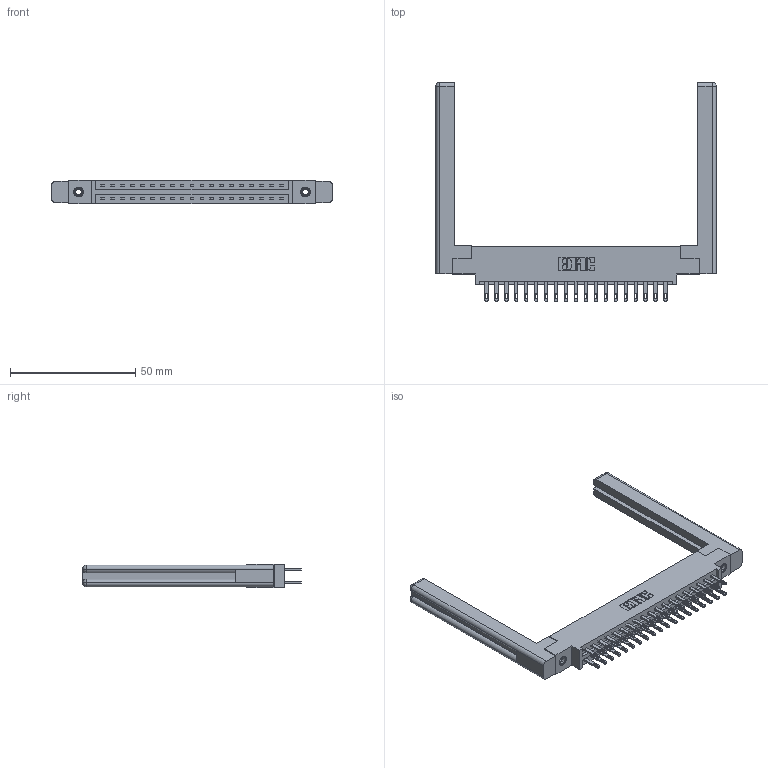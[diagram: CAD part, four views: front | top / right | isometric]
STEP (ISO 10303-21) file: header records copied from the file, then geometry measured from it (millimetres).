
FILE_DESCRIPTION (( 'STEP AP203' ), '1' );
FILE_NAME ('337-038-500-858.STEP', '2019-10-11T11:07:55', ( '' ), ( '' ), 'SwSTEP 2.0', 'SolidWorks 2016', '' );
FILE_SCHEMA (( 'CONFIG_CONTROL_DESIGN' ));
Length unit declared in the file: inch
Products named in the file (5): 337 Part_0.170 Offset - 0.156 Dia-TI; 337-038-500-858; 345-250-001_345-250-001-102; 345-292-001_345-293-100; 307-220-058
Assembly tree (43 placements, depth 2):
  337-038-500-858
    337 Part_0.170 Offset - 0.156 Dia-TI
    345-292-001_345-293-100  x38
    345-250-001_345-250-001-102  x2
    307-220-058  x2
Bounding box: 111.91 x 87.25 x 9.4 mm (x, y, z)
Volume: 18629 mm3; surface area: 18338.5 mm2
Topology: 43 solids, 43 shells, 2160 faces, 6491 edges, 4314 vertices
Faces by surface type: plane 1374, cylinder 762, cone 12, torus 12
Entity records: 20402 total; most frequent: CARTESIAN_POINT 3465, ORIENTED_EDGE 3340, DIRECTION 3006, EDGE_CURVE 1670, VECTOR 1490, LINE 1490, VERTEX_POINT 1106, AXIS2_PLACEMENT_3D 758
